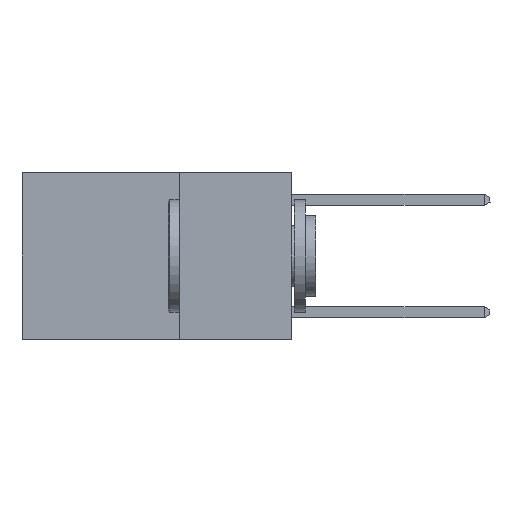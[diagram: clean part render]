
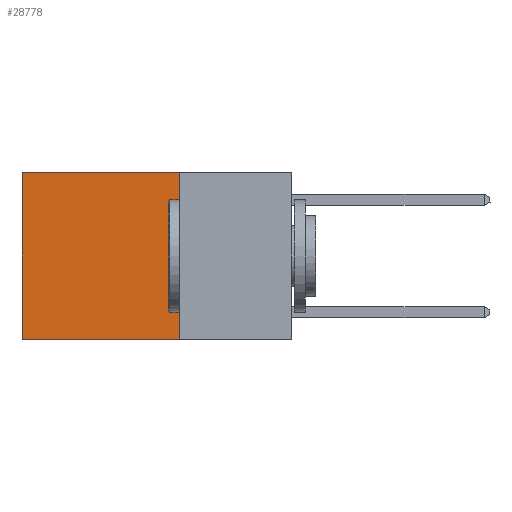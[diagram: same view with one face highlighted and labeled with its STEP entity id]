
A CAD part, left-side view. The second image highlights one B-rep face of the part: STEP entity #28778.
In plain terms, the highlighted planar face has unit normal (-1, 0, 0).
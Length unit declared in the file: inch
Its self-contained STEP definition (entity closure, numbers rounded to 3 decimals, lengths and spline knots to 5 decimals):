
#320 = CARTESIAN_POINT ( 'NONE',  ( 0.2625, 0.25, -0.37 ) ) ;
#1045 = CARTESIAN_POINT ( 'NONE',  ( 0.2625, 0.25, 0. ) ) ;
#1513 = FACE_OUTER_BOUND ( 'NONE', #6282, .T. ) ;
#2873 = VECTOR ( 'NONE', #14180, 39.37008 ) ;
#2920 = VECTOR ( 'NONE', #3353, 39.37008 ) ;
#3184 = CARTESIAN_POINT ( 'NONE',  ( 0.2625, 0.25, 0. ) ) ;
#3353 = DIRECTION ( 'NONE',  ( 0., 1., 0. ) ) ;
#3566 = AXIS2_PLACEMENT_3D ( 'NONE', #3184, #20627, #20293 ) ;
#6282 = EDGE_LOOP ( 'NONE', ( #9866, #9839, #29585, #15831 ) ) ;
#6811 = LINE ( 'NONE', #17077, #2873 ) ;
#7153 = LINE ( 'NONE', #1045, #8313 ) ;
#8313 = VECTOR ( 'NONE', #31114, 39.37008 ) ;
#9839 = ORIENTED_EDGE ( 'NONE', *, *, #19916, .F. ) ;
#9866 = ORIENTED_EDGE ( 'NONE', *, *, #10256, .T. ) ;
#10256 = EDGE_CURVE ( 'NONE', #27227, #31458, #23824, .T. ) ;
#14180 = DIRECTION ( 'NONE',  ( 0., 1., 0. ) ) ;
#14497 = VECTOR ( 'NONE', #20358, 39.37008 ) ;
#15831 = ORIENTED_EDGE ( 'NONE', *, *, #17702, .T. ) ;
#15897 = CARTESIAN_POINT ( 'NONE',  ( 0.2625, 0.25, 0. ) ) ;
#17077 = CARTESIAN_POINT ( 'NONE',  ( 0.2625, 0.25, -0.37 ) ) ;
#17702 = EDGE_CURVE ( 'NONE', #21140, #27227, #18552, .T. ) ;
#18552 = LINE ( 'NONE', #15897, #2920 ) ;
#19916 = EDGE_CURVE ( 'NONE', #26175, #31458, #6811, .T. ) ;
#20293 = DIRECTION ( 'NONE',  ( 0., 0., -1. ) ) ;
#20358 = DIRECTION ( 'NONE',  ( 0., 0., -1. ) ) ;
#20627 = DIRECTION ( 'NONE',  ( 1., 0., 0. ) ) ;
#21082 = CARTESIAN_POINT ( 'NONE',  ( 0.2625, 0.6, 0. ) ) ;
#21140 = VERTEX_POINT ( 'NONE', #23452 ) ;
#22064 = EDGE_CURVE ( 'NONE', #21140, #26175, #7153, .T. ) ;
#22760 = CARTESIAN_POINT ( 'NONE',  ( 0.2625, 0.6, 0. ) ) ;
#23452 = CARTESIAN_POINT ( 'NONE',  ( 0.2625, 0.25, 0. ) ) ;
#23824 = LINE ( 'NONE', #22760, #14497 ) ;
#25534 = PLANE ( 'NONE',  #3566 ) ;
#26175 = VERTEX_POINT ( 'NONE', #320 ) ;
#26252 = CARTESIAN_POINT ( 'NONE',  ( 0.2625, 0.6, -0.37 ) ) ;
#27227 = VERTEX_POINT ( 'NONE', #21082 ) ;
#28778 = ADVANCED_FACE ( 'NONE', ( #1513 ), #25534, .F. ) ;
#29585 = ORIENTED_EDGE ( 'NONE', *, *, #22064, .F. ) ;
#31114 = DIRECTION ( 'NONE',  ( 0., 0., -1. ) ) ;
#31458 = VERTEX_POINT ( 'NONE', #26252 ) ;
